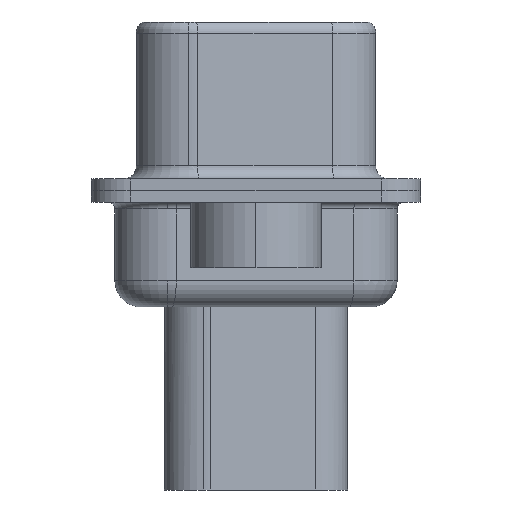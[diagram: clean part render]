
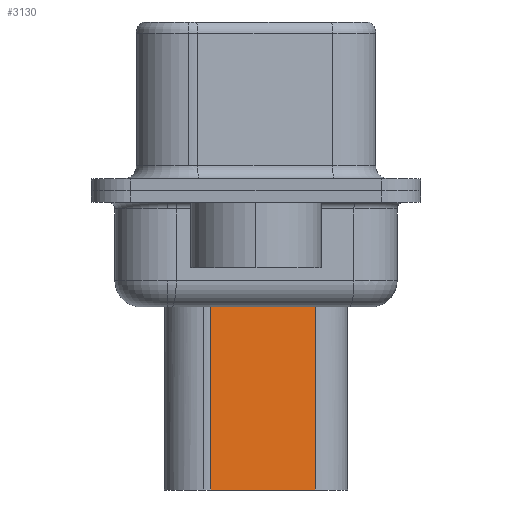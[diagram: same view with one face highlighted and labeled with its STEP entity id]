
A CAD part, left-side view. The second image highlights one B-rep face of the part: STEP entity #3130.
In plain terms, the highlighted planar face has unit normal (-0.985, -0.174, 0).
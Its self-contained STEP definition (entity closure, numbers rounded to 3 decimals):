
#90 = VECTOR ( 'NONE', #511, 1000. ) ;
#353 = DIRECTION ( 'NONE',  ( 0., 0., -1. ) ) ;
#511 = DIRECTION ( 'NONE',  ( -0.174, 0.985, 0. ) ) ;
#1814 = ORIENTED_EDGE ( 'NONE', *, *, #5447, .T. ) ;
#2290 = LINE ( 'NONE', #11714, #90 ) ;
#3130 = ADVANCED_FACE ( 'NONE', ( #5785 ), #5112, .T. ) ;
#3242 = ORIENTED_EDGE ( 'NONE', *, *, #9366, .F. ) ;
#3280 = DIRECTION ( 'NONE',  ( -0.985, -0.174, 0. ) ) ;
#3486 = VERTEX_POINT ( 'NONE', #6667 ) ;
#3631 = VERTEX_POINT ( 'NONE', #5524 ) ;
#3635 = VERTEX_POINT ( 'NONE', #9309 ) ;
#3761 = EDGE_LOOP ( 'NONE', ( #3242, #1814, #4468, #9106 ) ) ;
#4103 = VECTOR ( 'NONE', #12137, 1000. ) ;
#4468 = ORIENTED_EDGE ( 'NONE', *, *, #8406, .T. ) ;
#5051 = VECTOR ( 'NONE', #353, 1000. ) ;
#5112 = PLANE ( 'NONE',  #7030 ) ;
#5420 = CARTESIAN_POINT ( 'NONE',  ( 5.229, -2.26, -11.45 ) ) ;
#5447 = EDGE_CURVE ( 'NONE', #3635, #3631, #2290, .T. ) ;
#5491 = LINE ( 'NONE', #12131, #10205 ) ;
#5524 = CARTESIAN_POINT ( 'NONE',  ( 4.524, 1.74, -3.975 ) ) ;
#5785 = FACE_OUTER_BOUND ( 'NONE', #3761, .T. ) ;
#6667 = CARTESIAN_POINT ( 'NONE',  ( 4.524, 1.74, -11.45 ) ) ;
#7010 = CARTESIAN_POINT ( 'NONE',  ( 4.524, 1.74, -3.1 ) ) ;
#7030 = AXIS2_PLACEMENT_3D ( 'NONE', #7010, #3280, #9846 ) ;
#8002 = VERTEX_POINT ( 'NONE', #5420 ) ;
#8406 = EDGE_CURVE ( 'NONE', #3631, #3486, #10065, .T. ) ;
#8439 = CARTESIAN_POINT ( 'NONE',  ( 5.229, -2.26, -3.1 ) ) ;
#9106 = ORIENTED_EDGE ( 'NONE', *, *, #11993, .F. ) ;
#9123 = LINE ( 'NONE', #8439, #4103 ) ;
#9309 = CARTESIAN_POINT ( 'NONE',  ( 5.229, -2.26, -3.975 ) ) ;
#9366 = EDGE_CURVE ( 'NONE', #3635, #8002, #9123, .T. ) ;
#9846 = DIRECTION ( 'NONE',  ( 0.174, -0.985, 0. ) ) ;
#10065 = LINE ( 'NONE', #11571, #5051 ) ;
#10205 = VECTOR ( 'NONE', #11228, 1000. ) ;
#11228 = DIRECTION ( 'NONE',  ( -0.174, 0.985, 0. ) ) ;
#11571 = CARTESIAN_POINT ( 'NONE',  ( 4.524, 1.74, -3.1 ) ) ;
#11714 = CARTESIAN_POINT ( 'NONE',  ( 4.353, 2.709, -3.975 ) ) ;
#11993 = EDGE_CURVE ( 'NONE', #8002, #3486, #5491, .T. ) ;
#12131 = CARTESIAN_POINT ( 'NONE',  ( 4.524, 1.74, -11.45 ) ) ;
#12137 = DIRECTION ( 'NONE',  ( 0., 0., -1. ) ) ;
